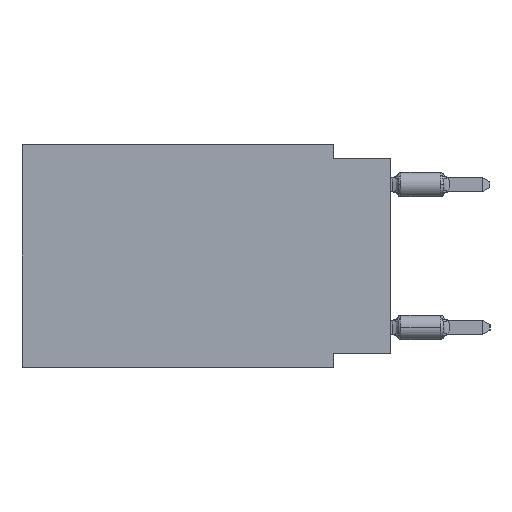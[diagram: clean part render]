
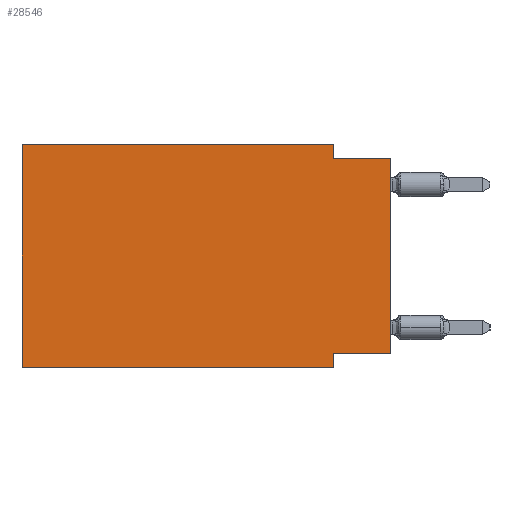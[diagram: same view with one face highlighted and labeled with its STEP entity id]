
A CAD part, left-side view. The second image highlights one B-rep face of the part: STEP entity #28546.
In plain terms, the highlighted planar face has unit normal (-1, 0, 0).
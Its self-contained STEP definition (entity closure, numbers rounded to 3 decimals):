
#840 = CARTESIAN_POINT ( 'NONE',  ( 0., 0., -0.635 ) ) ;
#2578 = VERTEX_POINT ( 'NONE', #63320 ) ;
#4802 = CARTESIAN_POINT ( 'NONE',  ( 0., 2.54, -9.906 ) ) ;
#5473 = LINE ( 'NONE', #45803, #46216 ) ;
#5494 = CARTESIAN_POINT ( 'NONE',  ( 0., 0., -9.271 ) ) ;
#5995 = EDGE_CURVE ( 'NONE', #41788, #56088, #5473, .T. ) ;
#6567 = ORIENTED_EDGE ( 'NONE', *, *, #42669, .F. ) ;
#7532 = ORIENTED_EDGE ( 'NONE', *, *, #34651, .F. ) ;
#9975 = LINE ( 'NONE', #29951, #62599 ) ;
#10066 = CARTESIAN_POINT ( 'NONE',  ( 0., 0., -0.635 ) ) ;
#10089 = DIRECTION ( 'NONE',  ( 0., 0., 1. ) ) ;
#13614 = VERTEX_POINT ( 'NONE', #62690 ) ;
#15212 = DIRECTION ( 'NONE',  ( 1., 0., 0. ) ) ;
#15620 = LINE ( 'NONE', #10066, #20498 ) ;
#18803 = DIRECTION ( 'NONE',  ( 0., 0., -1. ) ) ;
#18916 = CARTESIAN_POINT ( 'NONE',  ( 0., 2.54, 0. ) ) ;
#19067 = EDGE_CURVE ( 'NONE', #50299, #13614, #34194, .T. ) ;
#19799 = DIRECTION ( 'NONE',  ( 0., 0., -1. ) ) ;
#20498 = VECTOR ( 'NONE', #45784, 1000. ) ;
#20593 = VERTEX_POINT ( 'NONE', #43028 ) ;
#21767 = VECTOR ( 'NONE', #63534, 1000. ) ;
#23071 = VECTOR ( 'NONE', #40575, 1000. ) ;
#24702 = FACE_OUTER_BOUND ( 'NONE', #52333, .T. ) ;
#25016 = PLANE ( 'NONE',  #46816 ) ;
#25621 = DIRECTION ( 'NONE',  ( 0., 0., -1. ) ) ;
#28546 = ADVANCED_FACE ( 'NONE', ( #24702 ), #25016, .F. ) ;
#29508 = EDGE_CURVE ( 'NONE', #20593, #60351, #42598, .T. ) ;
#29951 = CARTESIAN_POINT ( 'NONE',  ( 0., 16.383, 0. ) ) ;
#30433 = VECTOR ( 'NONE', #42433, 1000. ) ;
#32744 = EDGE_CURVE ( 'NONE', #41788, #56617, #39936, .T. ) ;
#34194 = LINE ( 'NONE', #39448, #55855 ) ;
#34651 = EDGE_CURVE ( 'NONE', #20593, #2578, #36181, .T. ) ;
#35760 = CARTESIAN_POINT ( 'NONE',  ( 0., 0., -9.271 ) ) ;
#36181 = LINE ( 'NONE', #51941, #30433 ) ;
#39104 = ORIENTED_EDGE ( 'NONE', *, *, #5995, .T. ) ;
#39448 = CARTESIAN_POINT ( 'NONE',  ( 0., 2.54, 0. ) ) ;
#39936 = LINE ( 'NONE', #5494, #23071 ) ;
#40575 = DIRECTION ( 'NONE',  ( 0., 1., 0. ) ) ;
#41099 = ORIENTED_EDGE ( 'NONE', *, *, #56388, .F. ) ;
#41580 = ORIENTED_EDGE ( 'NONE', *, *, #32744, .F. ) ;
#41788 = VERTEX_POINT ( 'NONE', #35760 ) ;
#42433 = DIRECTION ( 'NONE',  ( 0., 0., 1. ) ) ;
#42598 = LINE ( 'NONE', #62582, #21767 ) ;
#42669 = EDGE_CURVE ( 'NONE', #13614, #56088, #15620, .T. ) ;
#43028 = CARTESIAN_POINT ( 'NONE',  ( 0., 16.383, -9.906 ) ) ;
#45557 = EDGE_CURVE ( 'NONE', #2578, #50299, #9975, .T. ) ;
#45784 = DIRECTION ( 'NONE',  ( 0., -1., 0. ) ) ;
#45803 = CARTESIAN_POINT ( 'NONE',  ( 0., 0., 0. ) ) ;
#46216 = VECTOR ( 'NONE', #10089, 1000. ) ;
#46816 = AXIS2_PLACEMENT_3D ( 'NONE', #64379, #15212, #19799 ) ;
#49960 = DIRECTION ( 'NONE',  ( 0., -1., 0. ) ) ;
#50299 = VERTEX_POINT ( 'NONE', #18916 ) ;
#51941 = CARTESIAN_POINT ( 'NONE',  ( 0., 16.383, 0. ) ) ;
#52333 = EDGE_LOOP ( 'NONE', ( #39104, #6567, #58410, #61518, #7532, #60750, #41099, #41580 ) ) ;
#55145 = CARTESIAN_POINT ( 'NONE',  ( 0., 2.54, -9.906 ) ) ;
#55855 = VECTOR ( 'NONE', #18803, 1000. ) ;
#56088 = VERTEX_POINT ( 'NONE', #840 ) ;
#56388 = EDGE_CURVE ( 'NONE', #56617, #60351, #60706, .T. ) ;
#56617 = VERTEX_POINT ( 'NONE', #64195 ) ;
#58410 = ORIENTED_EDGE ( 'NONE', *, *, #19067, .F. ) ;
#60351 = VERTEX_POINT ( 'NONE', #4802 ) ;
#60706 = LINE ( 'NONE', #55145, #63376 ) ;
#60750 = ORIENTED_EDGE ( 'NONE', *, *, #29508, .T. ) ;
#61518 = ORIENTED_EDGE ( 'NONE', *, *, #45557, .F. ) ;
#62582 = CARTESIAN_POINT ( 'NONE',  ( 0., 16.383, -9.906 ) ) ;
#62599 = VECTOR ( 'NONE', #49960, 1000. ) ;
#62690 = CARTESIAN_POINT ( 'NONE',  ( 0., 2.54, -0.635 ) ) ;
#63320 = CARTESIAN_POINT ( 'NONE',  ( 0., 16.383, 0. ) ) ;
#63376 = VECTOR ( 'NONE', #25621, 1000. ) ;
#63534 = DIRECTION ( 'NONE',  ( 0., -1., 0. ) ) ;
#64195 = CARTESIAN_POINT ( 'NONE',  ( 0., 2.54, -9.271 ) ) ;
#64379 = CARTESIAN_POINT ( 'NONE',  ( 0., 16.383, 0. ) ) ;
